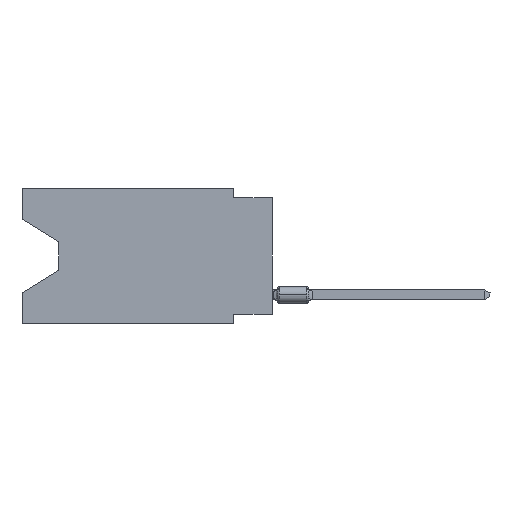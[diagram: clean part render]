
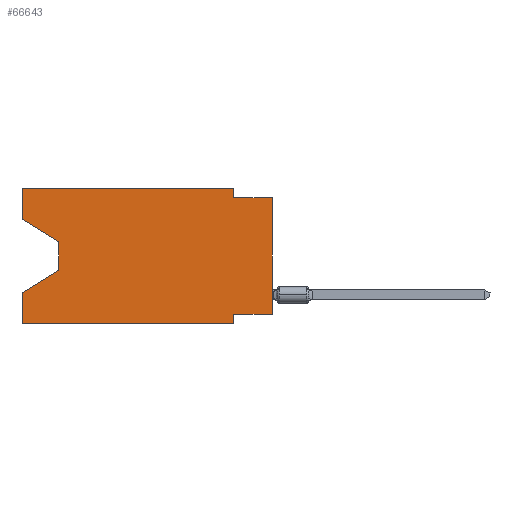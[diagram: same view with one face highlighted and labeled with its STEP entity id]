
A CAD part, left-side view. The second image highlights one B-rep face of the part: STEP entity #66643.
In plain terms, the highlighted planar face has unit normal (-1, 0, 0).
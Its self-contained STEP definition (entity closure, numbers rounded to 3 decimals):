
#138 = CARTESIAN_POINT ( 'NONE',  ( 0., 13.97, -3.505 ) ) ;
#1787 = EDGE_CURVE ( 'NONE', #76595, #25827, #80069, .T. ) ;
#4581 = LINE ( 'NONE', #12622, #19174 ) ;
#5009 = CARTESIAN_POINT ( 'NONE',  ( 0., 2.54, 0. ) ) ;
#6331 = EDGE_CURVE ( 'NONE', #55154, #76595, #9368, .T. ) ;
#7840 = CARTESIAN_POINT ( 'NONE',  ( 0., 0., -0.635 ) ) ;
#8926 = DIRECTION ( 'NONE',  ( 0., 0., -1. ) ) ;
#9368 = LINE ( 'NONE', #39643, #47469 ) ;
#11589 = VECTOR ( 'NONE', #32049, 1000. ) ;
#12622 = CARTESIAN_POINT ( 'NONE',  ( 0., 0., 0. ) ) ;
#14242 = EDGE_CURVE ( 'NONE', #39633, #91833, #93046, .T. ) ;
#14287 = CARTESIAN_POINT ( 'NONE',  ( 0., 16.383, -6.852 ) ) ;
#14648 = CARTESIAN_POINT ( 'NONE',  ( 0., 16.383, 0. ) ) ;
#15132 = FACE_OUTER_BOUND ( 'NONE', #84755, .T. ) ;
#15207 = AXIS2_PLACEMENT_3D ( 'NONE', #14648, #61013, #82693 ) ;
#16839 = ORIENTED_EDGE ( 'NONE', *, *, #32024, .F. ) ;
#19174 = VECTOR ( 'NONE', #74116, 1000. ) ;
#19512 = ORIENTED_EDGE ( 'NONE', *, *, #54905, .T. ) ;
#19670 = VECTOR ( 'NONE', #21731, 1000. ) ;
#20987 = VERTEX_POINT ( 'NONE', #138 ) ;
#21731 = DIRECTION ( 'NONE',  ( 0., -0.855, -0.519 ) ) ;
#21810 = LINE ( 'NONE', #98407, #91491 ) ;
#21856 = CARTESIAN_POINT ( 'NONE',  ( 0., 2.54, -8.89 ) ) ;
#23570 = CARTESIAN_POINT ( 'NONE',  ( 0., 2.54, -8.89 ) ) ;
#25797 = EDGE_CURVE ( 'NONE', #20987, #65690, #41693, .T. ) ;
#25827 = VERTEX_POINT ( 'NONE', #64371 ) ;
#26301 = CARTESIAN_POINT ( 'NONE',  ( 0., 13.97, -5.385 ) ) ;
#27242 = VECTOR ( 'NONE', #48759, 1000. ) ;
#28958 = CARTESIAN_POINT ( 'NONE',  ( 0., 0., -0.635 ) ) ;
#29843 = EDGE_CURVE ( 'NONE', #60737, #55154, #79353, .T. ) ;
#30474 = EDGE_CURVE ( 'NONE', #60737, #20987, #88314, .T. ) ;
#31387 = VERTEX_POINT ( 'NONE', #14287 ) ;
#32024 = EDGE_CURVE ( 'NONE', #33777, #91833, #92609, .T. ) ;
#32049 = DIRECTION ( 'NONE',  ( 0., -1., 0. ) ) ;
#32316 = CARTESIAN_POINT ( 'NONE',  ( 0., 16.383, -2.038 ) ) ;
#32582 = ORIENTED_EDGE ( 'NONE', *, *, #53837, .T. ) ;
#33527 = CARTESIAN_POINT ( 'NONE',  ( 0., 16.383, 0. ) ) ;
#33777 = VERTEX_POINT ( 'NONE', #96001 ) ;
#33955 = VECTOR ( 'NONE', #84986, 1000. ) ;
#34858 = LINE ( 'NONE', #26301, #93145 ) ;
#35005 = ORIENTED_EDGE ( 'NONE', *, *, #6331, .F. ) ;
#37349 = PLANE ( 'NONE',  #15207 ) ;
#39633 = VERTEX_POINT ( 'NONE', #56850 ) ;
#39643 = CARTESIAN_POINT ( 'NONE',  ( 0., 16.383, 0. ) ) ;
#40669 = VECTOR ( 'NONE', #75406, 1000. ) ;
#41693 = LINE ( 'NONE', #80483, #27242 ) ;
#42129 = VECTOR ( 'NONE', #49633, 1000. ) ;
#44509 = CARTESIAN_POINT ( 'NONE',  ( 0., 0., -8.255 ) ) ;
#46474 = EDGE_CURVE ( 'NONE', #25827, #96415, #91536, .T. ) ;
#47133 = ORIENTED_EDGE ( 'NONE', *, *, #98356, .F. ) ;
#47469 = VECTOR ( 'NONE', #87496, 1000. ) ;
#48759 = DIRECTION ( 'NONE',  ( 0., 0., -1. ) ) ;
#49633 = DIRECTION ( 'NONE',  ( 0., 0., 1. ) ) ;
#50259 = ORIENTED_EDGE ( 'NONE', *, *, #53524, .F. ) ;
#52756 = CARTESIAN_POINT ( 'NONE',  ( 0., 16.383, -8.89 ) ) ;
#53524 = EDGE_CURVE ( 'NONE', #39633, #31387, #21810, .T. ) ;
#53837 = EDGE_CURVE ( 'NONE', #70150, #96415, #4581, .T. ) ;
#54905 = EDGE_CURVE ( 'NONE', #65690, #31387, #34858, .T. ) ;
#55154 = VERTEX_POINT ( 'NONE', #91743 ) ;
#56850 = CARTESIAN_POINT ( 'NONE',  ( 0., 16.383, -8.89 ) ) ;
#57124 = VECTOR ( 'NONE', #8926, 1000. ) ;
#59861 = ORIENTED_EDGE ( 'NONE', *, *, #1787, .F. ) ;
#60293 = LINE ( 'NONE', #66868, #40669 ) ;
#60737 = VERTEX_POINT ( 'NONE', #32316 ) ;
#61013 = DIRECTION ( 'NONE',  ( 1., 0., 0. ) ) ;
#62720 = ORIENTED_EDGE ( 'NONE', *, *, #46474, .F. ) ;
#64371 = CARTESIAN_POINT ( 'NONE',  ( 0., 2.54, -0.635 ) ) ;
#65690 = VERTEX_POINT ( 'NONE', #80965 ) ;
#66643 = ADVANCED_FACE ( 'NONE', ( #15132 ), #37349, .F. ) ;
#66868 = CARTESIAN_POINT ( 'NONE',  ( 0., 0., -8.255 ) ) ;
#68595 = CARTESIAN_POINT ( 'NONE',  ( 0., 16.383, -2.038 ) ) ;
#70150 = VERTEX_POINT ( 'NONE', #44509 ) ;
#72812 = VECTOR ( 'NONE', #78571, 1000. ) ;
#74116 = DIRECTION ( 'NONE',  ( 0., 0., 1. ) ) ;
#75406 = DIRECTION ( 'NONE',  ( 0., 1., 0. ) ) ;
#76595 = VERTEX_POINT ( 'NONE', #5009 ) ;
#78571 = DIRECTION ( 'NONE',  ( 0., 0., -1. ) ) ;
#79353 = LINE ( 'NONE', #33527, #42129 ) ;
#79554 = CARTESIAN_POINT ( 'NONE',  ( 0., 2.54, 0. ) ) ;
#80069 = LINE ( 'NONE', #79554, #72812 ) ;
#80437 = ORIENTED_EDGE ( 'NONE', *, *, #30474, .T. ) ;
#80483 = CARTESIAN_POINT ( 'NONE',  ( 0., 13.97, -3.505 ) ) ;
#80965 = CARTESIAN_POINT ( 'NONE',  ( 0., 13.97, -5.385 ) ) ;
#81796 = DIRECTION ( 'NONE',  ( 0., 0., 1. ) ) ;
#82693 = DIRECTION ( 'NONE',  ( 0., 0., -1. ) ) ;
#84755 = EDGE_LOOP ( 'NONE', ( #80437, #98872, #19512, #50259, #85032, #16839, #47133, #32582, #62720, #59861, #35005, #91629 ) ) ;
#84986 = DIRECTION ( 'NONE',  ( 0., -1., 0. ) ) ;
#85032 = ORIENTED_EDGE ( 'NONE', *, *, #14242, .T. ) ;
#87496 = DIRECTION ( 'NONE',  ( 0., -1., 0. ) ) ;
#88314 = LINE ( 'NONE', #68595, #19670 ) ;
#91491 = VECTOR ( 'NONE', #81796, 1000. ) ;
#91536 = LINE ( 'NONE', #7840, #11589 ) ;
#91629 = ORIENTED_EDGE ( 'NONE', *, *, #29843, .F. ) ;
#91743 = CARTESIAN_POINT ( 'NONE',  ( 0., 16.383, 0. ) ) ;
#91833 = VERTEX_POINT ( 'NONE', #21856 ) ;
#92609 = LINE ( 'NONE', #23570, #57124 ) ;
#93046 = LINE ( 'NONE', #52756, #33955 ) ;
#93145 = VECTOR ( 'NONE', #95340, 1000. ) ;
#95340 = DIRECTION ( 'NONE',  ( 0., 0.855, -0.519 ) ) ;
#96001 = CARTESIAN_POINT ( 'NONE',  ( 0., 2.54, -8.255 ) ) ;
#96415 = VERTEX_POINT ( 'NONE', #28958 ) ;
#98356 = EDGE_CURVE ( 'NONE', #70150, #33777, #60293, .T. ) ;
#98407 = CARTESIAN_POINT ( 'NONE',  ( 0., 16.383, 0. ) ) ;
#98872 = ORIENTED_EDGE ( 'NONE', *, *, #25797, .T. ) ;
